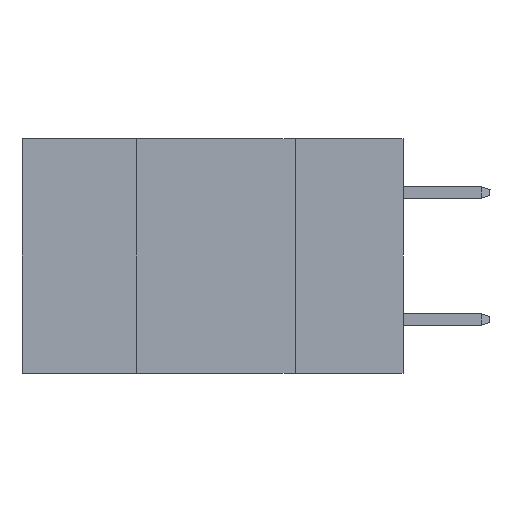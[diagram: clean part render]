
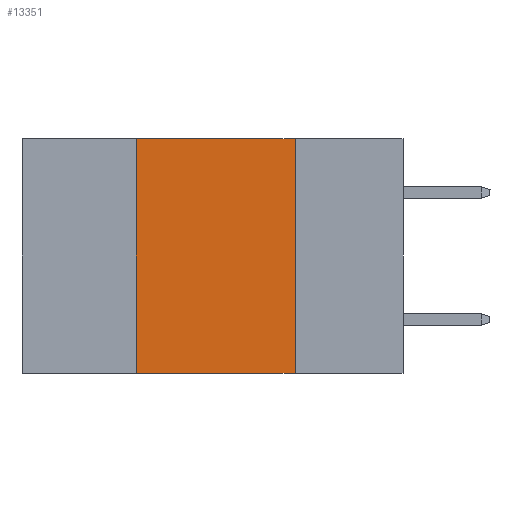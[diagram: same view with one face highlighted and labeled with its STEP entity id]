
A CAD part, left-side view. The second image highlights one B-rep face of the part: STEP entity #13351.
In plain terms, the highlighted planar face has unit normal (-1, 0, 0).
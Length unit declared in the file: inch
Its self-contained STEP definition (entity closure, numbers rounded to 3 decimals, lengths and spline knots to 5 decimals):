
#911 = DIRECTION ( 'NONE',  ( 0., -1., 0. ) ) ;
#926 = DIRECTION ( 'NONE',  ( 0., 0., -1. ) ) ;
#992 = AXIS2_PLACEMENT_3D ( 'NONE', #18232, #10974, #926 ) ;
#2162 = CARTESIAN_POINT ( 'NONE',  ( 0., 0.42, 0. ) ) ;
#4732 = VECTOR ( 'NONE', #5088, 39.37008 ) ;
#5026 = LINE ( 'NONE', #8978, #9418 ) ;
#5088 = DIRECTION ( 'NONE',  ( 0., 0., 1. ) ) ;
#5903 = EDGE_CURVE ( 'NONE', #13015, #18008, #15203, .T. ) ;
#6594 = PLANE ( 'NONE',  #992 ) ;
#7731 = EDGE_CURVE ( 'NONE', #17950, #13015, #16486, .T. ) ;
#8109 = CARTESIAN_POINT ( 'NONE',  ( 0., 0.6, 0. ) ) ;
#8196 = CARTESIAN_POINT ( 'NONE',  ( 0., 0.42, -0.37 ) ) ;
#8390 = VECTOR ( 'NONE', #10544, 39.37008 ) ;
#8724 = EDGE_LOOP ( 'NONE', ( #16326, #18214, #15575, #8866 ) ) ;
#8866 = ORIENTED_EDGE ( 'NONE', *, *, #11915, .T. ) ;
#8978 = CARTESIAN_POINT ( 'NONE',  ( 0., 0.6, -0.37 ) ) ;
#9418 = VECTOR ( 'NONE', #15211, 39.37008 ) ;
#9439 = CARTESIAN_POINT ( 'NONE',  ( 0., 0.17, -0.37 ) ) ;
#10544 = DIRECTION ( 'NONE',  ( 0., 0., -1. ) ) ;
#10974 = DIRECTION ( 'NONE',  ( 1., 0., 0. ) ) ;
#11915 = EDGE_CURVE ( 'NONE', #13154, #18008, #5026, .T. ) ;
#12177 = CARTESIAN_POINT ( 'NONE',  ( 0., 0.17, 0. ) ) ;
#13015 = VERTEX_POINT ( 'NONE', #16455 ) ;
#13154 = VERTEX_POINT ( 'NONE', #8196 ) ;
#13323 = VECTOR ( 'NONE', #911, 39.37008 ) ;
#13351 = ADVANCED_FACE ( 'NONE', ( #17058 ), #6594, .F. ) ;
#15184 = LINE ( 'NONE', #2162, #4732 ) ;
#15203 = LINE ( 'NONE', #12177, #8390 ) ;
#15211 = DIRECTION ( 'NONE',  ( 0., -1., 0. ) ) ;
#15575 = ORIENTED_EDGE ( 'NONE', *, *, #17533, .F. ) ;
#16215 = CARTESIAN_POINT ( 'NONE',  ( 0., 0.42, 0. ) ) ;
#16326 = ORIENTED_EDGE ( 'NONE', *, *, #5903, .F. ) ;
#16455 = CARTESIAN_POINT ( 'NONE',  ( 0., 0.17, 0. ) ) ;
#16486 = LINE ( 'NONE', #8109, #13323 ) ;
#17058 = FACE_OUTER_BOUND ( 'NONE', #8724, .T. ) ;
#17533 = EDGE_CURVE ( 'NONE', #13154, #17950, #15184, .T. ) ;
#17950 = VERTEX_POINT ( 'NONE', #16215 ) ;
#18008 = VERTEX_POINT ( 'NONE', #9439 ) ;
#18214 = ORIENTED_EDGE ( 'NONE', *, *, #7731, .F. ) ;
#18232 = CARTESIAN_POINT ( 'NONE',  ( 0., 0.6, 0. ) ) ;
